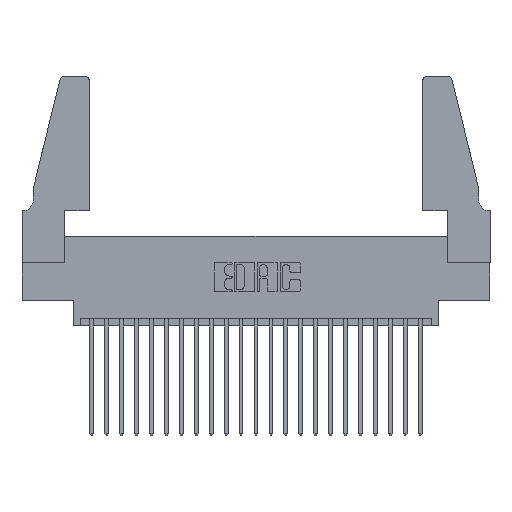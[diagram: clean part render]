
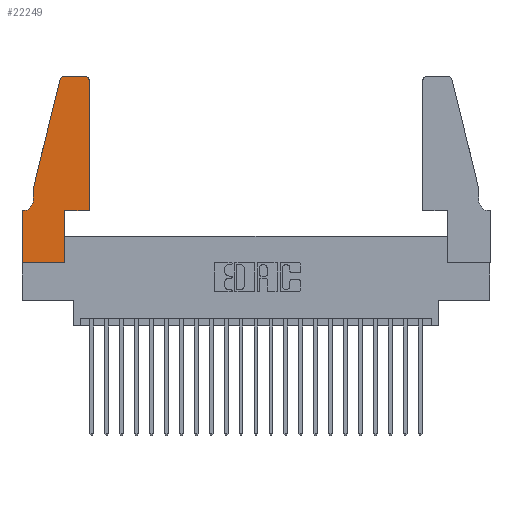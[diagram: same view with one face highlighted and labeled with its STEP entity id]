
A CAD part, top view. The second image highlights one B-rep face of the part: STEP entity #22249.
In plain terms, the highlighted planar face has unit normal (0, 0, 1).
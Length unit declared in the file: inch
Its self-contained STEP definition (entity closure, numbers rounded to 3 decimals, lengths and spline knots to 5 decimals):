
#16 = DIRECTION ( 'NONE',  ( 1., 0., 0. ) ) ;
#542 = EDGE_CURVE ( 'NONE', #7271, #12492, #4206, .T. ) ;
#1078 = DIRECTION ( 'NONE',  ( 0., -1., 0. ) ) ;
#1091 = DIRECTION ( 'NONE',  ( 1., 0., 0. ) ) ;
#1185 = CIRCLE ( 'NONE', #12559, 0.07 ) ;
#1449 = ORIENTED_EDGE ( 'NONE', *, *, #10006, .T. ) ;
#1916 = CARTESIAN_POINT ( 'NONE',  ( 0.0755, 0.35, 0.37 ) ) ;
#2067 = EDGE_CURVE ( 'NONE', #16872, #17802, #1185, .T. ) ;
#2232 = VECTOR ( 'NONE', #19492, 39.37008 ) ;
#2291 = VECTOR ( 'NONE', #6279, 39.37008 ) ;
#2818 = DIRECTION ( 'NONE',  ( 0., 0., 1. ) ) ;
#2840 = LINE ( 'NONE', #10931, #2232 ) ;
#2979 = CIRCLE ( 'NONE', #15529, 0.03 ) ;
#3060 = CARTESIAN_POINT ( 'NONE',  ( 0.0755, 0.5, 0.37 ) ) ;
#3101 = CARTESIAN_POINT ( 'NONE',  ( 0.4505, 1.22, 0.37 ) ) ;
#3162 = CARTESIAN_POINT ( 'NONE',  ( 0.25487, 1.22718, 0.37 ) ) ;
#3432 = CIRCLE ( 'NONE', #8137, 0.03 ) ;
#3520 = ORIENTED_EDGE ( 'NONE', *, *, #21089, .T. ) ;
#3594 = CARTESIAN_POINT ( 'NONE',  ( 0.4505, 0.35, 0.37 ) ) ;
#3641 = EDGE_CURVE ( 'NONE', #15171, #21188, #13236, .T. ) ;
#3943 = VERTEX_POINT ( 'NONE', #21237 ) ;
#4061 = LINE ( 'NONE', #4239, #17538 ) ;
#4206 = LINE ( 'NONE', #10146, #7359 ) ;
#4239 = CARTESIAN_POINT ( 'NONE',  ( 0.2865, 0.35, 0.37 ) ) ;
#4339 = CARTESIAN_POINT ( 'NONE',  ( 0.2865, 0.35, 0.37 ) ) ;
#4401 = CARTESIAN_POINT ( 'NONE',  ( 0.4205, 1.25, 0.37 ) ) ;
#4557 = EDGE_CURVE ( 'NONE', #3943, #15171, #9141, .T. ) ;
#4593 = CARTESIAN_POINT ( 'NONE',  ( 0.0755, 0.5, 0.37 ) ) ;
#5230 = LINE ( 'NONE', #3060, #15161 ) ;
#5422 = DIRECTION ( 'NONE',  ( 0., 1., 0. ) ) ;
#5566 = DIRECTION ( 'NONE',  ( -1., 0., 0. ) ) ;
#5616 = DIRECTION ( 'NONE',  ( 0., 0., -1. ) ) ;
#6279 = DIRECTION ( 'NONE',  ( 1., 0., 0. ) ) ;
#7210 = LINE ( 'NONE', #13302, #2291 ) ;
#7242 = ORIENTED_EDGE ( 'NONE', *, *, #2067, .T. ) ;
#7271 = VERTEX_POINT ( 'NONE', #4401 ) ;
#7359 = VECTOR ( 'NONE', #10192, 39.37008 ) ;
#7450 = PLANE ( 'NONE',  #11505 ) ;
#7520 = VERTEX_POINT ( 'NONE', #3162 ) ;
#7729 = CARTESIAN_POINT ( 'NONE',  ( 0.284, 1.25, 0.37 ) ) ;
#8137 = AXIS2_PLACEMENT_3D ( 'NONE', #13517, #2818, #15261 ) ;
#8529 = CARTESIAN_POINT ( 'NONE',  ( 0.0055, 0.42, 0.37 ) ) ;
#8938 = DIRECTION ( 'NONE',  ( 0., 0., 1. ) ) ;
#9141 = LINE ( 'NONE', #21213, #13726 ) ;
#9279 = EDGE_CURVE ( 'NONE', #21188, #10662, #4061, .T. ) ;
#9305 = DIRECTION ( 'NONE',  ( -1., 0., 0. ) ) ;
#10006 = EDGE_CURVE ( 'NONE', #10662, #12374, #7210, .T. ) ;
#10026 = ORIENTED_EDGE ( 'NONE', *, *, #3641, .T. ) ;
#10146 = CARTESIAN_POINT ( 'NONE',  ( 0.2605, 1.25, 0.37 ) ) ;
#10192 = DIRECTION ( 'NONE',  ( -1., 0., 0. ) ) ;
#10662 = VERTEX_POINT ( 'NONE', #4339 ) ;
#10931 = CARTESIAN_POINT ( 'NONE',  ( 0.0755, 0.5, 0.37 ) ) ;
#11004 = DIRECTION ( 'NONE',  ( 0., 0., 1. ) ) ;
#11142 = VECTOR ( 'NONE', #5422, 39.37008 ) ;
#11505 = AXIS2_PLACEMENT_3D ( 'NONE', #19559, #11004, #16 ) ;
#11657 = LINE ( 'NONE', #3594, #11142 ) ;
#11776 = FACE_OUTER_BOUND ( 'NONE', #17032, .T. ) ;
#12374 = VERTEX_POINT ( 'NONE', #21247 ) ;
#12492 = VERTEX_POINT ( 'NONE', #7729 ) ;
#12559 = AXIS2_PLACEMENT_3D ( 'NONE', #8529, #5616, #5566 ) ;
#13236 = LINE ( 'NONE', #15436, #21810 ) ;
#13302 = CARTESIAN_POINT ( 'NONE',  ( 0.4505, 0.35, 0.37 ) ) ;
#13517 = CARTESIAN_POINT ( 'NONE',  ( 0.284, 1.22, 0.37 ) ) ;
#13726 = VECTOR ( 'NONE', #14324, 39.37008 ) ;
#14194 = EDGE_CURVE ( 'NONE', #12374, #16486, #11657, .T. ) ;
#14324 = DIRECTION ( 'NONE',  ( 0., -1., 0. ) ) ;
#14711 = EDGE_CURVE ( 'NONE', #21884, #16872, #5230, .T. ) ;
#14822 = CARTESIAN_POINT ( 'NONE',  ( 0.0755, 0.42, 0.37 ) ) ;
#14843 = DIRECTION ( 'NONE',  ( 0., 1., 0. ) ) ;
#15161 = VECTOR ( 'NONE', #1078, 39.37008 ) ;
#15170 = ORIENTED_EDGE ( 'NONE', *, *, #9279, .T. ) ;
#15171 = VERTEX_POINT ( 'NONE', #22081 ) ;
#15261 = DIRECTION ( 'NONE',  ( 1., 0., 0. ) ) ;
#15437 = ORIENTED_EDGE ( 'NONE', *, *, #16177, .T. ) ;
#15436 = CARTESIAN_POINT ( 'NONE',  ( 0., 0., 0.37 ) ) ;
#15529 = AXIS2_PLACEMENT_3D ( 'NONE', #19244, #8938, #20957 ) ;
#16177 = EDGE_CURVE ( 'NONE', #7520, #21884, #2840, .T. ) ;
#16393 = CARTESIAN_POINT ( 'NONE',  ( 0.2865, 0., 0.37 ) ) ;
#16486 = VERTEX_POINT ( 'NONE', #3101 ) ;
#16872 = VERTEX_POINT ( 'NONE', #14822 ) ;
#17032 = EDGE_LOOP ( 'NONE', ( #22374, #18891, #15437, #19956, #7242, #3520, #18104, #10026, #15170, #1449, #21318, #22395 ) ) ;
#17538 = VECTOR ( 'NONE', #14843, 39.37008 ) ;
#17779 = LINE ( 'NONE', #1916, #21771 ) ;
#17802 = VERTEX_POINT ( 'NONE', #18619 ) ;
#18104 = ORIENTED_EDGE ( 'NONE', *, *, #4557, .T. ) ;
#18619 = CARTESIAN_POINT ( 'NONE',  ( 0.0055, 0.35, 0.37 ) ) ;
#18672 = EDGE_CURVE ( 'NONE', #16486, #7271, #2979, .T. ) ;
#18891 = ORIENTED_EDGE ( 'NONE', *, *, #21381, .T. ) ;
#19244 = CARTESIAN_POINT ( 'NONE',  ( 0.4205, 1.22, 0.37 ) ) ;
#19492 = DIRECTION ( 'NONE',  ( -0.239, -0.971, 0. ) ) ;
#19559 = CARTESIAN_POINT ( 'NONE',  ( 0., 0.35, 0.37 ) ) ;
#19956 = ORIENTED_EDGE ( 'NONE', *, *, #14711, .T. ) ;
#20957 = DIRECTION ( 'NONE',  ( 1., 0., 0. ) ) ;
#21089 = EDGE_CURVE ( 'NONE', #17802, #3943, #17779, .T. ) ;
#21188 = VERTEX_POINT ( 'NONE', #16393 ) ;
#21213 = CARTESIAN_POINT ( 'NONE',  ( 0., 0., 0.37 ) ) ;
#21237 = CARTESIAN_POINT ( 'NONE',  ( 0., 0.35, 0.37 ) ) ;
#21247 = CARTESIAN_POINT ( 'NONE',  ( 0.4505, 0.35, 0.37 ) ) ;
#21318 = ORIENTED_EDGE ( 'NONE', *, *, #14194, .T. ) ;
#21381 = EDGE_CURVE ( 'NONE', #12492, #7520, #3432, .T. ) ;
#21771 = VECTOR ( 'NONE', #9305, 39.37008 ) ;
#21810 = VECTOR ( 'NONE', #1091, 39.37008 ) ;
#21884 = VERTEX_POINT ( 'NONE', #4593 ) ;
#22081 = CARTESIAN_POINT ( 'NONE',  ( 0., 0., 0.37 ) ) ;
#22249 = ADVANCED_FACE ( 'NONE', ( #11776 ), #7450, .T. ) ;
#22374 = ORIENTED_EDGE ( 'NONE', *, *, #542, .T. ) ;
#22395 = ORIENTED_EDGE ( 'NONE', *, *, #18672, .T. ) ;
